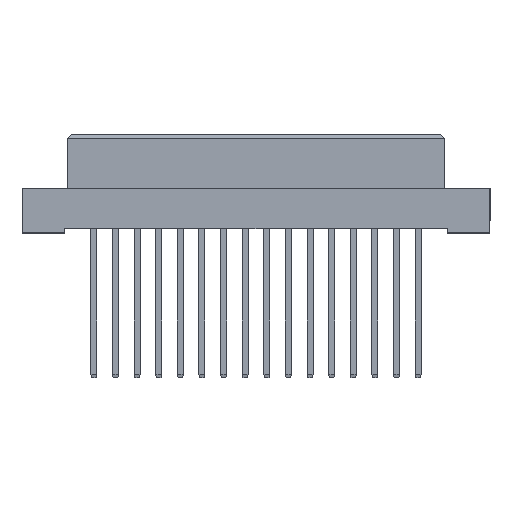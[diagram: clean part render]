
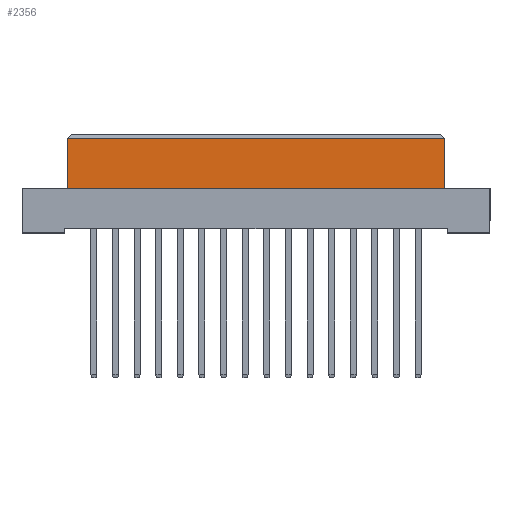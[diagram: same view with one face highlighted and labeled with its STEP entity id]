
A CAD part, top view. The second image highlights one B-rep face of the part: STEP entity #2356.
In plain terms, the highlighted planar face has unit normal (0, 0, 1).
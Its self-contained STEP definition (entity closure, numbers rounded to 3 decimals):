
#1116 = LINE ( 'NONE', #15427, #7417 ) ;
#1443 = DIRECTION ( 'NONE',  ( 1., 0., 0. ) ) ;
#2356 = ADVANCED_FACE ( 'NONE', ( #3336 ), #19529, .T. ) ;
#2667 = VECTOR ( 'NONE', #1443, 1000. ) ;
#2817 = CARTESIAN_POINT ( 'NONE',  ( 22.2, -6.4, 4.25 ) ) ;
#3001 = CARTESIAN_POINT ( 'NONE',  ( -22.2, -6.4, 4.25 ) ) ;
#3047 = EDGE_LOOP ( 'NONE', ( #11890, #12019, #9095, #5341 ) ) ;
#3336 = FACE_OUTER_BOUND ( 'NONE', #3047, .T. ) ;
#3956 = CARTESIAN_POINT ( 'NONE',  ( 22.2, -0.5, 4.25 ) ) ;
#5126 = DIRECTION ( 'NONE',  ( 1., 0., 0. ) ) ;
#5216 = CARTESIAN_POINT ( 'NONE',  ( 22.2, -6.4, 4.25 ) ) ;
#5251 = VERTEX_POINT ( 'NONE', #6114 ) ;
#5341 = ORIENTED_EDGE ( 'NONE', *, *, #10981, .T. ) ;
#5584 = VERTEX_POINT ( 'NONE', #3956 ) ;
#5756 = DIRECTION ( 'NONE',  ( -1., 0., 0. ) ) ;
#6114 = CARTESIAN_POINT ( 'NONE',  ( 22.2, -6.4, 4.25 ) ) ;
#6547 = VERTEX_POINT ( 'NONE', #15691 ) ;
#7417 = VECTOR ( 'NONE', #5756, 1000. ) ;
#7934 = DIRECTION ( 'NONE',  ( 0., 1., 0. ) ) ;
#9095 = ORIENTED_EDGE ( 'NONE', *, *, #19983, .F. ) ;
#9230 = DIRECTION ( 'NONE',  ( 0., 1., 0. ) ) ;
#9717 = CARTESIAN_POINT ( 'NONE',  ( -22.2, -6.4, 4.25 ) ) ;
#9760 = DIRECTION ( 'NONE',  ( 0., 0., 1. ) ) ;
#10981 = EDGE_CURVE ( 'NONE', #12506, #5251, #11131, .T. ) ;
#11131 = LINE ( 'NONE', #15872, #2667 ) ;
#11890 = ORIENTED_EDGE ( 'NONE', *, *, #14132, .T. ) ;
#12019 = ORIENTED_EDGE ( 'NONE', *, *, #12272, .T. ) ;
#12272 = EDGE_CURVE ( 'NONE', #5584, #6547, #1116, .T. ) ;
#12506 = VERTEX_POINT ( 'NONE', #3001 ) ;
#14132 = EDGE_CURVE ( 'NONE', #5251, #5584, #17228, .T. ) ;
#15427 = CARTESIAN_POINT ( 'NONE',  ( -22.2, -0.5, 4.25 ) ) ;
#15691 = CARTESIAN_POINT ( 'NONE',  ( -22.2, -0.5, 4.25 ) ) ;
#15872 = CARTESIAN_POINT ( 'NONE',  ( 22.2, -6.4, 4.25 ) ) ;
#17228 = LINE ( 'NONE', #2817, #20750 ) ;
#17421 = VECTOR ( 'NONE', #7934, 1000. ) ;
#17605 = AXIS2_PLACEMENT_3D ( 'NONE', #5216, #9760, #5126 ) ;
#19188 = LINE ( 'NONE', #9717, #17421 ) ;
#19529 = PLANE ( 'NONE',  #17605 ) ;
#19983 = EDGE_CURVE ( 'NONE', #12506, #6547, #19188, .T. ) ;
#20750 = VECTOR ( 'NONE', #9230, 1000. ) ;
